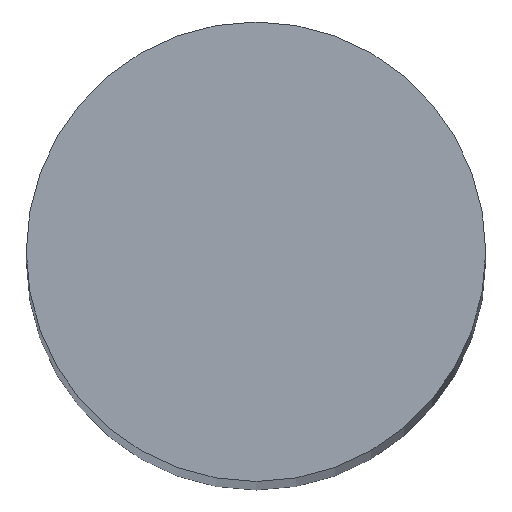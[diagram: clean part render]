
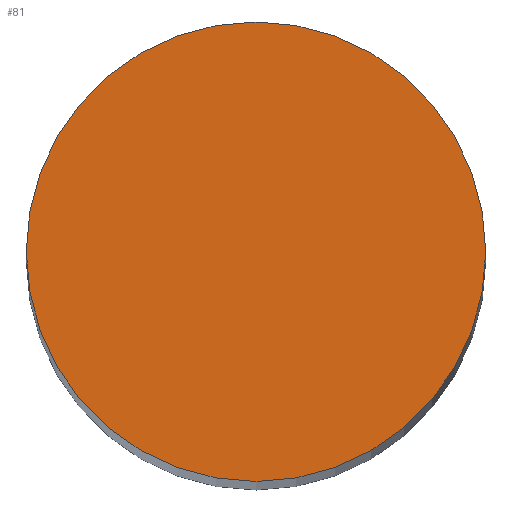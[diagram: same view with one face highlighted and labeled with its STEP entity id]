
A CAD part, top view. The second image highlights one B-rep face of the part: STEP entity #81.
In plain terms, the highlighted planar face has unit normal (0, 0, 1).
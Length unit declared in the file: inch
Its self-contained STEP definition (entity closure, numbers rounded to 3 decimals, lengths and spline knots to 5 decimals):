
#6 = CARTESIAN_POINT ( 'NONE',  ( 0.05906, 0., 1.00551 ) ) ;
#17 = CARTESIAN_POINT ( 'NONE',  ( -0.05906, 0., 1.00551 ) ) ;
#20 = CARTESIAN_POINT ( 'NONE',  ( 0., 0., 1.00551 ) ) ;
#22 = DIRECTION ( 'NONE',  ( 1., 0., 0. ) ) ;
#26 = DIRECTION ( 'NONE',  ( 0., 0., 1. ) ) ;
#28 = PLANE ( 'NONE',  #78 ) ;
#46 = DIRECTION ( 'NONE',  ( 1., 0., 0. ) ) ;
#51 = DIRECTION ( 'NONE',  ( 0., 0., 1. ) ) ;
#54 = CARTESIAN_POINT ( 'NONE',  ( 0., 0., 1.00551 ) ) ;
#60 = DIRECTION ( 'NONE',  ( 0., 0., 1. ) ) ;
#67 = DIRECTION ( 'NONE',  ( 1., 0., 0. ) ) ;
#70 = AXIS2_PLACEMENT_3D ( 'NONE', #20, #26, #67 ) ;
#73 = CARTESIAN_POINT ( 'NONE',  ( 0., 0., 1.00551 ) ) ;
#78 = AXIS2_PLACEMENT_3D ( 'NONE', #73, #51, #46 ) ;
#80 = AXIS2_PLACEMENT_3D ( 'NONE', #54, #60, #22 ) ;
#81 = ADVANCED_FACE ( 'NONE', ( #115 ), #28, .T. ) ;
#106 = CIRCLE ( 'NONE', #70, 0.05906 ) ;
#114 = CIRCLE ( 'NONE', #80, 0.05906 ) ;
#115 = FACE_OUTER_BOUND ( 'NONE', #133, .T. ) ;
#119 = EDGE_CURVE ( 'NONE', #145, #136, #114, .T. ) ;
#123 = ORIENTED_EDGE ( 'NONE', *, *, #142, .T. ) ;
#124 = ORIENTED_EDGE ( 'NONE', *, *, #119, .T. ) ;
#133 = EDGE_LOOP ( 'NONE', ( #124, #123 ) ) ;
#136 = VERTEX_POINT ( 'NONE', #17 ) ;
#142 = EDGE_CURVE ( 'NONE', #136, #145, #106, .T. ) ;
#145 = VERTEX_POINT ( 'NONE', #6 ) ;
